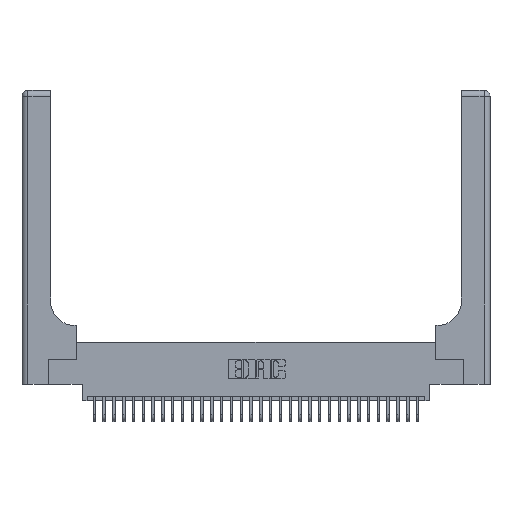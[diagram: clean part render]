
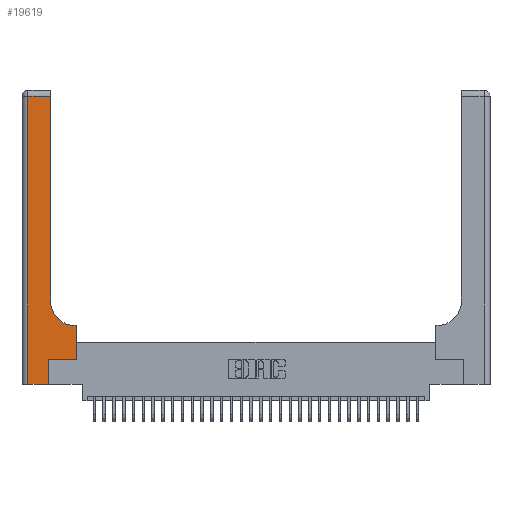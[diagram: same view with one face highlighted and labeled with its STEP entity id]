
A CAD part, top view. The second image highlights one B-rep face of the part: STEP entity #19619.
In plain terms, the highlighted planar face has unit normal (0, 0, 1).
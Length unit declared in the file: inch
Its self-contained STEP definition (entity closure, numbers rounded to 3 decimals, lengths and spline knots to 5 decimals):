
#145 = CARTESIAN_POINT ( 'NONE',  ( 0.269, 0., 0.37 ) ) ;
#1761 = CARTESIAN_POINT ( 'NONE',  ( 0.06, 0., 0.37 ) ) ;
#4016 = VERTEX_POINT ( 'NONE', #13465 ) ;
#4294 = LINE ( 'NONE', #22524, #29456 ) ;
#4517 = LINE ( 'NONE', #27478, #9167 ) ;
#4754 = CARTESIAN_POINT ( 'NONE',  ( 0.5415, 0.6, 0.37 ) ) ;
#4935 = DIRECTION ( 'NONE',  ( 0., -1., 0. ) ) ;
#6876 = LINE ( 'NONE', #20937, #24495 ) ;
#6927 = VERTEX_POINT ( 'NONE', #14239 ) ;
#7108 = CARTESIAN_POINT ( 'NONE',  ( 0.06, 2.94, 0.37 ) ) ;
#7938 = DIRECTION ( 'NONE',  ( 1., 0., 0. ) ) ;
#8024 = ORIENTED_EDGE ( 'NONE', *, *, #9440, .T. ) ;
#8183 = CARTESIAN_POINT ( 'NONE',  ( 0.269, 0.25, 0.37 ) ) ;
#8625 = VECTOR ( 'NONE', #7938, 39.37008 ) ;
#9084 = ORIENTED_EDGE ( 'NONE', *, *, #22597, .T. ) ;
#9167 = VECTOR ( 'NONE', #24794, 39.37008 ) ;
#9337 = VERTEX_POINT ( 'NONE', #1761 ) ;
#9440 = EDGE_CURVE ( 'NONE', #17217, #6927, #25776, .T. ) ;
#9729 = ORIENTED_EDGE ( 'NONE', *, *, #24890, .T. ) ;
#10135 = CARTESIAN_POINT ( 'NONE',  ( 0.06, 3., 0.37 ) ) ;
#10553 = VECTOR ( 'NONE', #20867, 39.37008 ) ;
#11837 = DIRECTION ( 'NONE',  ( 0., 1., 0. ) ) ;
#12071 = DIRECTION ( 'NONE',  ( -1., 0., 0. ) ) ;
#13037 = DIRECTION ( 'NONE',  ( 0., 1., 0. ) ) ;
#13465 = CARTESIAN_POINT ( 'NONE',  ( 0.2915, 0.85, 0.37 ) ) ;
#13895 = VERTEX_POINT ( 'NONE', #7108 ) ;
#14016 = ORIENTED_EDGE ( 'NONE', *, *, #21975, .T. ) ;
#14239 = CARTESIAN_POINT ( 'NONE',  ( 0.5585, 0.25, 0.37 ) ) ;
#14302 = CARTESIAN_POINT ( 'NONE',  ( 0.269, 0., 0.37 ) ) ;
#15485 = VECTOR ( 'NONE', #11837, 39.37008 ) ;
#15721 = CARTESIAN_POINT ( 'NONE',  ( 0.2915, 3., 0.37 ) ) ;
#16023 = ORIENTED_EDGE ( 'NONE', *, *, #20850, .T. ) ;
#16531 = DIRECTION ( 'NONE',  ( 1., 0., 0. ) ) ;
#17143 = DIRECTION ( 'NONE',  ( -1., 0., 0. ) ) ;
#17217 = VERTEX_POINT ( 'NONE', #26024 ) ;
#18202 = VERTEX_POINT ( 'NONE', #145 ) ;
#19459 = EDGE_CURVE ( 'NONE', #22571, #4016, #32070, .T. ) ;
#19619 = ADVANCED_FACE ( 'NONE', ( #28702 ), #33702, .F. ) ;
#20678 = ORIENTED_EDGE ( 'NONE', *, *, #19459, .T. ) ;
#20763 = LINE ( 'NONE', #15721, #34601 ) ;
#20850 = EDGE_CURVE ( 'NONE', #34581, #13895, #4294, .T. ) ;
#20867 = DIRECTION ( 'NONE',  ( 0., 1., 0. ) ) ;
#20937 = CARTESIAN_POINT ( 'NONE',  ( 0., 0., 0.37 ) ) ;
#21428 = EDGE_CURVE ( 'NONE', #18202, #17217, #23436, .T. ) ;
#21805 = CARTESIAN_POINT ( 'NONE',  ( 0.5415, 0.85, 0.37 ) ) ;
#21975 = EDGE_CURVE ( 'NONE', #4016, #34581, #20763, .T. ) ;
#22524 = CARTESIAN_POINT ( 'NONE',  ( 0., 2.94, 0.37 ) ) ;
#22571 = VERTEX_POINT ( 'NONE', #4754 ) ;
#22597 = EDGE_CURVE ( 'NONE', #9337, #18202, #6876, .T. ) ;
#22676 = CARTESIAN_POINT ( 'NONE',  ( 0.5585, 0.25, 0.37 ) ) ;
#22958 = DIRECTION ( 'NONE',  ( 0., 0., -1. ) ) ;
#23436 = LINE ( 'NONE', #14302, #15485 ) ;
#24495 = VECTOR ( 'NONE', #34056, 39.37008 ) ;
#24794 = DIRECTION ( 'NONE',  ( -1., 0., 0. ) ) ;
#24890 = EDGE_CURVE ( 'NONE', #6927, #25935, #25603, .T. ) ;
#25603 = LINE ( 'NONE', #22676, #10553 ) ;
#25646 = CARTESIAN_POINT ( 'NONE',  ( 0.5585, 0.6, 0.37 ) ) ;
#25776 = LINE ( 'NONE', #8183, #8625 ) ;
#25935 = VERTEX_POINT ( 'NONE', #25646 ) ;
#26024 = CARTESIAN_POINT ( 'NONE',  ( 0.269, 0.25, 0.37 ) ) ;
#26076 = EDGE_LOOP ( 'NONE', ( #14016, #16023, #31673, #9084, #29502, #8024, #9729, #27066, #20678 ) ) ;
#26222 = EDGE_CURVE ( 'NONE', #25935, #22571, #4517, .T. ) ;
#26270 = VECTOR ( 'NONE', #4935, 39.37008 ) ;
#27040 = EDGE_CURVE ( 'NONE', #13895, #9337, #27955, .T. ) ;
#27066 = ORIENTED_EDGE ( 'NONE', *, *, #26222, .T. ) ;
#27478 = CARTESIAN_POINT ( 'NONE',  ( 0.2915, 0.6, 0.37 ) ) ;
#27781 = AXIS2_PLACEMENT_3D ( 'NONE', #21805, #29874, #16531 ) ;
#27955 = LINE ( 'NONE', #10135, #26270 ) ;
#28702 = FACE_OUTER_BOUND ( 'NONE', #26076, .T. ) ;
#29456 = VECTOR ( 'NONE', #17143, 39.37008 ) ;
#29502 = ORIENTED_EDGE ( 'NONE', *, *, #21428, .T. ) ;
#29874 = DIRECTION ( 'NONE',  ( 0., 0., -1. ) ) ;
#30717 = AXIS2_PLACEMENT_3D ( 'NONE', #31142, #22958, #12071 ) ;
#31142 = CARTESIAN_POINT ( 'NONE',  ( 0., 3., 0.37 ) ) ;
#31576 = CARTESIAN_POINT ( 'NONE',  ( 0.2915, 2.94, 0.37 ) ) ;
#31673 = ORIENTED_EDGE ( 'NONE', *, *, #27040, .T. ) ;
#32070 = CIRCLE ( 'NONE', #27781, 0.25 ) ;
#33702 = PLANE ( 'NONE',  #30717 ) ;
#34056 = DIRECTION ( 'NONE',  ( 1., 0., 0. ) ) ;
#34581 = VERTEX_POINT ( 'NONE', #31576 ) ;
#34601 = VECTOR ( 'NONE', #13037, 39.37008 ) ;
